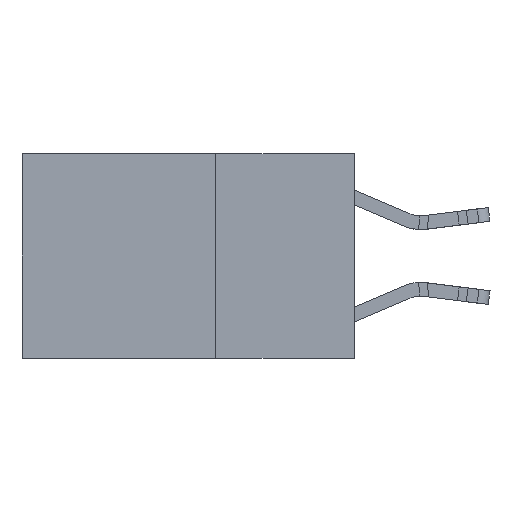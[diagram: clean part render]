
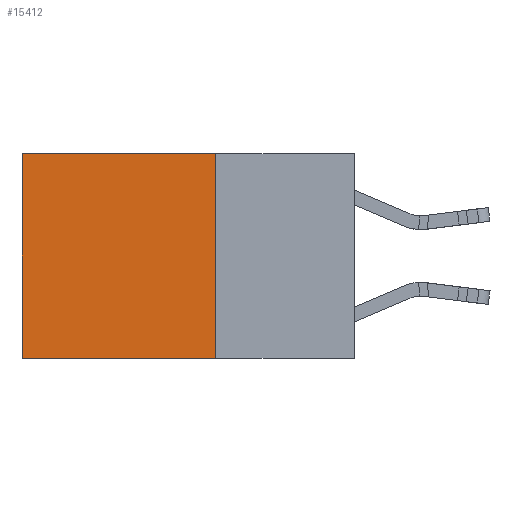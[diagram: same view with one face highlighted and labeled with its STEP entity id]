
A CAD part, left-side view. The second image highlights one B-rep face of the part: STEP entity #15412.
In plain terms, the highlighted planar face has unit normal (-1, 0, 0).
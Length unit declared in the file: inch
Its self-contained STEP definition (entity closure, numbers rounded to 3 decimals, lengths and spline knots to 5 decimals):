
#1017 = ORIENTED_EDGE ( 'NONE', *, *, #13168, .T. ) ;
#1137 = ORIENTED_EDGE ( 'NONE', *, *, #6048, .T. ) ;
#1436 = DIRECTION ( 'NONE',  ( 1., 0., 0. ) ) ;
#1845 = CARTESIAN_POINT ( 'NONE',  ( 0.2625, 0.25, 0. ) ) ;
#2176 = LINE ( 'NONE', #12937, #26982 ) ;
#2880 = VERTEX_POINT ( 'NONE', #5721 ) ;
#3267 = CARTESIAN_POINT ( 'NONE',  ( 0.2625, 0.6, -0.37 ) ) ;
#3322 = CARTESIAN_POINT ( 'NONE',  ( 0.2625, 0.25, 0. ) ) ;
#5052 = CARTESIAN_POINT ( 'NONE',  ( 0.2625, 0.25, 0. ) ) ;
#5356 = VERTEX_POINT ( 'NONE', #15868 ) ;
#5721 = CARTESIAN_POINT ( 'NONE',  ( 0.2625, 0.25, -0.37 ) ) ;
#6048 = EDGE_CURVE ( 'NONE', #5356, #28353, #12271, .T. ) ;
#7248 = EDGE_CURVE ( 'NONE', #2880, #23303, #22582, .T. ) ;
#7722 = ORIENTED_EDGE ( 'NONE', *, *, #11046, .F. ) ;
#8837 = FACE_OUTER_BOUND ( 'NONE', #18673, .T. ) ;
#10117 = CARTESIAN_POINT ( 'NONE',  ( 0.2625, 0.6, 0. ) ) ;
#10381 = CARTESIAN_POINT ( 'NONE',  ( 0.2625, 0.25, -0.37 ) ) ;
#10458 = VECTOR ( 'NONE', #16795, 39.37008 ) ;
#10791 = ORIENTED_EDGE ( 'NONE', *, *, #7248, .F. ) ;
#11046 = EDGE_CURVE ( 'NONE', #5356, #2880, #22071, .T. ) ;
#12271 = LINE ( 'NONE', #3322, #10458 ) ;
#12937 = CARTESIAN_POINT ( 'NONE',  ( 0.2625, 0.6, 0. ) ) ;
#13168 = EDGE_CURVE ( 'NONE', #28353, #23303, #2176, .T. ) ;
#15412 = ADVANCED_FACE ( 'NONE', ( #8837 ), #28992, .F. ) ;
#15868 = CARTESIAN_POINT ( 'NONE',  ( 0.2625, 0.25, 0. ) ) ;
#16689 = DIRECTION ( 'NONE',  ( 0., 0., -1. ) ) ;
#16795 = DIRECTION ( 'NONE',  ( 0., 1., 0. ) ) ;
#17119 = DIRECTION ( 'NONE',  ( 0., 1., 0. ) ) ;
#18673 = EDGE_LOOP ( 'NONE', ( #1017, #10791, #7722, #1137 ) ) ;
#18991 = VECTOR ( 'NONE', #17119, 39.37008 ) ;
#21842 = DIRECTION ( 'NONE',  ( 0., 0., -1. ) ) ;
#22071 = LINE ( 'NONE', #5052, #23518 ) ;
#22109 = DIRECTION ( 'NONE',  ( 0., 0., -1. ) ) ;
#22582 = LINE ( 'NONE', #10381, #18991 ) ;
#23303 = VERTEX_POINT ( 'NONE', #3267 ) ;
#23518 = VECTOR ( 'NONE', #16689, 39.37008 ) ;
#25302 = AXIS2_PLACEMENT_3D ( 'NONE', #1845, #1436, #22109 ) ;
#26982 = VECTOR ( 'NONE', #21842, 39.37008 ) ;
#28353 = VERTEX_POINT ( 'NONE', #10117 ) ;
#28992 = PLANE ( 'NONE',  #25302 ) ;
